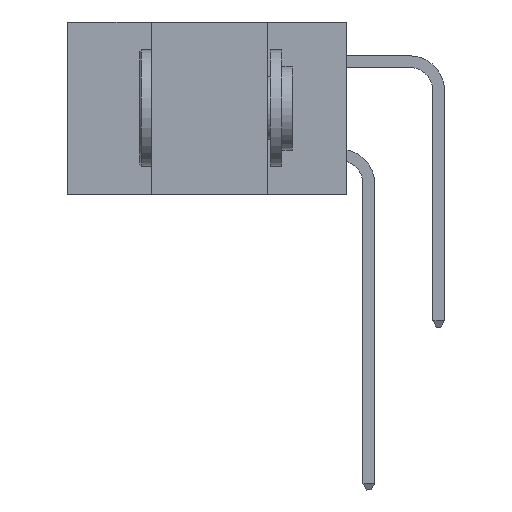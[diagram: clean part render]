
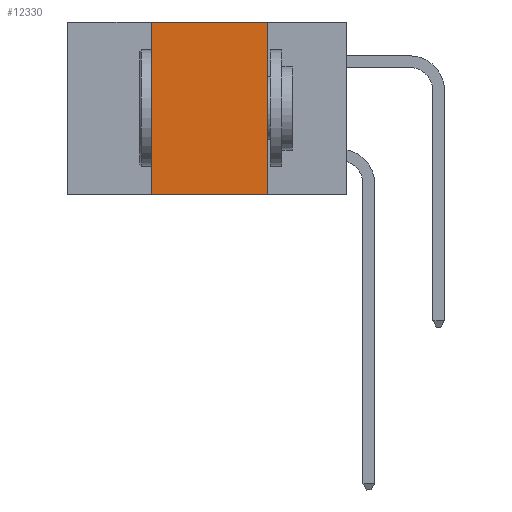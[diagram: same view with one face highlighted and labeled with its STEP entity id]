
A CAD part, left-side view. The second image highlights one B-rep face of the part: STEP entity #12330.
In plain terms, the highlighted planar face has unit normal (-1, 0, 0).
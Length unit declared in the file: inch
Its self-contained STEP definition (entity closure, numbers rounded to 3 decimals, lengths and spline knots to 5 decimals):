
#924 = PLANE ( 'NONE',  #7155 ) ;
#1605 = VERTEX_POINT ( 'NONE', #5592 ) ;
#2007 = EDGE_CURVE ( 'NONE', #18179, #1605, #7714, .T. ) ;
#3184 = EDGE_LOOP ( 'NONE', ( #12553, #19771, #12575, #16742 ) ) ;
#3793 = VECTOR ( 'NONE', #5603, 39.37008 ) ;
#4181 = DIRECTION ( 'NONE',  ( 0., -1., 0. ) ) ;
#5592 = CARTESIAN_POINT ( 'NONE',  ( 0., 0.17, 0. ) ) ;
#5603 = DIRECTION ( 'NONE',  ( 0., 0., 1. ) ) ;
#6049 = LINE ( 'NONE', #14590, #11948 ) ;
#6301 = DIRECTION ( 'NONE',  ( 1., 0., 0. ) ) ;
#6415 = FACE_OUTER_BOUND ( 'NONE', #3184, .T. ) ;
#6494 = CARTESIAN_POINT ( 'NONE',  ( 0., 0.42, -0.37 ) ) ;
#6636 = DIRECTION ( 'NONE',  ( 0., -1., 0. ) ) ;
#7155 = AXIS2_PLACEMENT_3D ( 'NONE', #16648, #6301, #18342 ) ;
#7714 = LINE ( 'NONE', #14200, #20840 ) ;
#8058 = DIRECTION ( 'NONE',  ( 0., 0., -1. ) ) ;
#8973 = CARTESIAN_POINT ( 'NONE',  ( 0., 0.42, 0. ) ) ;
#9493 = LINE ( 'NONE', #8973, #3793 ) ;
#10677 = CARTESIAN_POINT ( 'NONE',  ( 0., 0.17, -0.37 ) ) ;
#11483 = VERTEX_POINT ( 'NONE', #10677 ) ;
#11948 = VECTOR ( 'NONE', #4181, 39.37008 ) ;
#12330 = ADVANCED_FACE ( 'NONE', ( #6415 ), #924, .F. ) ;
#12553 = ORIENTED_EDGE ( 'NONE', *, *, #20690, .F. ) ;
#12575 = ORIENTED_EDGE ( 'NONE', *, *, #20391, .F. ) ;
#14200 = CARTESIAN_POINT ( 'NONE',  ( 0., 0.6, 0. ) ) ;
#14590 = CARTESIAN_POINT ( 'NONE',  ( 0., 0.6, -0.37 ) ) ;
#15433 = VERTEX_POINT ( 'NONE', #6494 ) ;
#16648 = CARTESIAN_POINT ( 'NONE',  ( 0., 0.6, 0. ) ) ;
#16686 = CARTESIAN_POINT ( 'NONE',  ( 0., 0.17, 0. ) ) ;
#16742 = ORIENTED_EDGE ( 'NONE', *, *, #20514, .T. ) ;
#17317 = CARTESIAN_POINT ( 'NONE',  ( 0., 0.42, 0. ) ) ;
#18179 = VERTEX_POINT ( 'NONE', #17317 ) ;
#18342 = DIRECTION ( 'NONE',  ( 0., 0., -1. ) ) ;
#18404 = VECTOR ( 'NONE', #8058, 39.37008 ) ;
#18946 = LINE ( 'NONE', #16686, #18404 ) ;
#19771 = ORIENTED_EDGE ( 'NONE', *, *, #2007, .F. ) ;
#20391 = EDGE_CURVE ( 'NONE', #15433, #18179, #9493, .T. ) ;
#20514 = EDGE_CURVE ( 'NONE', #15433, #11483, #6049, .T. ) ;
#20690 = EDGE_CURVE ( 'NONE', #1605, #11483, #18946, .T. ) ;
#20840 = VECTOR ( 'NONE', #6636, 39.37008 ) ;
